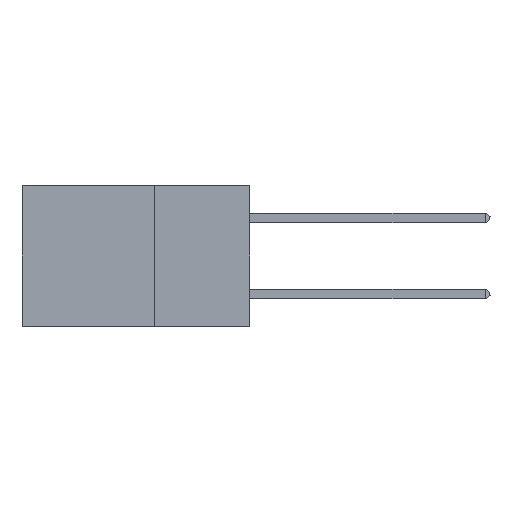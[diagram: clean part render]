
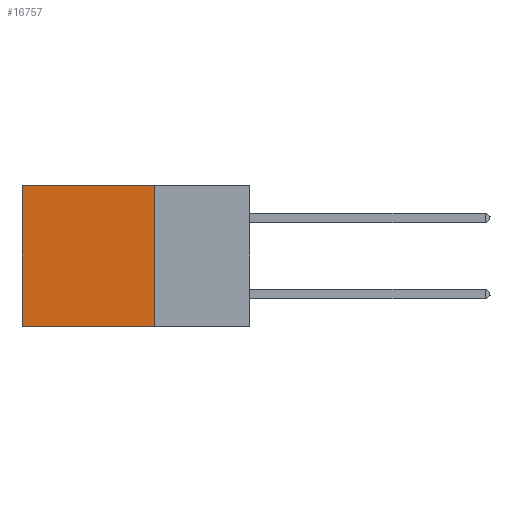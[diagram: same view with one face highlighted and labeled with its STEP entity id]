
A CAD part, left-side view. The second image highlights one B-rep face of the part: STEP entity #16757.
In plain terms, the highlighted planar face has unit normal (-1, 0, 0).
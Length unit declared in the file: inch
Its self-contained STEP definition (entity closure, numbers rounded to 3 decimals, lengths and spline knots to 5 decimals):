
#3417 = CARTESIAN_POINT ( 'NONE',  ( 0.2875, 0.25, 0. ) ) ;
#4228 = VERTEX_POINT ( 'NONE', #34291 ) ;
#4241 = FACE_OUTER_BOUND ( 'NONE', #28942, .T. ) ;
#4509 = LINE ( 'NONE', #26212, #36916 ) ;
#5746 = EDGE_CURVE ( 'NONE', #33970, #4228, #4509, .T. ) ;
#6220 = LINE ( 'NONE', #20066, #29945 ) ;
#7734 = DIRECTION ( 'NONE',  ( 0., 1., 0. ) ) ;
#11982 = AXIS2_PLACEMENT_3D ( 'NONE', #3417, #37048, #31094 ) ;
#13124 = CARTESIAN_POINT ( 'NONE',  ( 0.2875, 0.25, 0. ) ) ;
#13818 = ORIENTED_EDGE ( 'NONE', *, *, #22419, .F. ) ;
#15990 = VECTOR ( 'NONE', #16047, 39.37008 ) ;
#16047 = DIRECTION ( 'NONE',  ( 0., 0., -1. ) ) ;
#16757 = ADVANCED_FACE ( 'NONE', ( #4241 ), #37302, .F. ) ;
#16810 = LINE ( 'NONE', #13124, #37094 ) ;
#17718 = ORIENTED_EDGE ( 'NONE', *, *, #24172, .T. ) ;
#20066 = CARTESIAN_POINT ( 'NONE',  ( 0.2875, 0.25, -0.37 ) ) ;
#20622 = ORIENTED_EDGE ( 'NONE', *, *, #32579, .F. ) ;
#22419 = EDGE_CURVE ( 'NONE', #39372, #4228, #6220, .T. ) ;
#24172 = EDGE_CURVE ( 'NONE', #29303, #33970, #16810, .T. ) ;
#25317 = DIRECTION ( 'NONE',  ( 0., 1., 0. ) ) ;
#26212 = CARTESIAN_POINT ( 'NONE',  ( 0.2875, 0.6, 0. ) ) ;
#28319 = CARTESIAN_POINT ( 'NONE',  ( 0.2875, 0.25, 0. ) ) ;
#28942 = EDGE_LOOP ( 'NONE', ( #32548, #13818, #20622, #17718 ) ) ;
#28982 = CARTESIAN_POINT ( 'NONE',  ( 0.2875, 0.6, 0. ) ) ;
#29015 = CARTESIAN_POINT ( 'NONE',  ( 0.2875, 0.25, 0. ) ) ;
#29303 = VERTEX_POINT ( 'NONE', #29015 ) ;
#29945 = VECTOR ( 'NONE', #7734, 39.37008 ) ;
#31094 = DIRECTION ( 'NONE',  ( 0., 0., -1. ) ) ;
#32024 = DIRECTION ( 'NONE',  ( 0., 0., -1. ) ) ;
#32548 = ORIENTED_EDGE ( 'NONE', *, *, #5746, .T. ) ;
#32579 = EDGE_CURVE ( 'NONE', #29303, #39372, #39649, .T. ) ;
#33970 = VERTEX_POINT ( 'NONE', #28982 ) ;
#34291 = CARTESIAN_POINT ( 'NONE',  ( 0.2875, 0.6, -0.37 ) ) ;
#36916 = VECTOR ( 'NONE', #32024, 39.37008 ) ;
#37048 = DIRECTION ( 'NONE',  ( 1., 0., 0. ) ) ;
#37094 = VECTOR ( 'NONE', #25317, 39.37008 ) ;
#37302 = PLANE ( 'NONE',  #11982 ) ;
#39372 = VERTEX_POINT ( 'NONE', #39385 ) ;
#39385 = CARTESIAN_POINT ( 'NONE',  ( 0.2875, 0.25, -0.37 ) ) ;
#39649 = LINE ( 'NONE', #28319, #15990 ) ;
